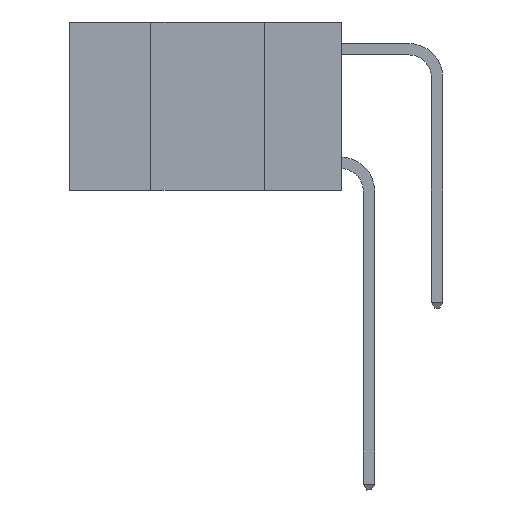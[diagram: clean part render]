
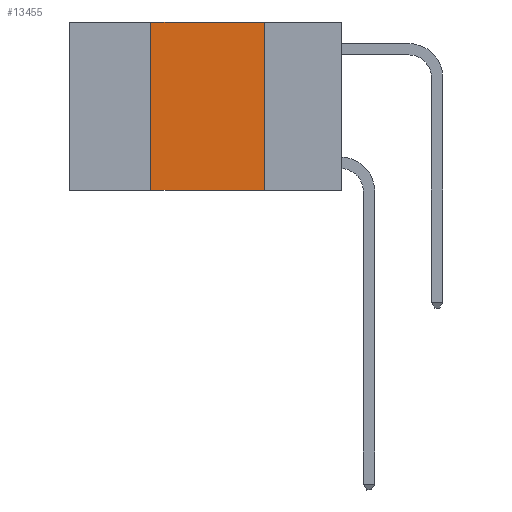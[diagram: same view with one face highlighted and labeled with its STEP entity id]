
A CAD part, left-side view. The second image highlights one B-rep face of the part: STEP entity #13455.
In plain terms, the highlighted planar face has unit normal (-1, 0, 0).
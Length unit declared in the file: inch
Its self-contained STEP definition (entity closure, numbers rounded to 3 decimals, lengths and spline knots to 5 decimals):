
#366 = LINE ( 'NONE', #11684, #16784 ) ;
#1702 = ORIENTED_EDGE ( 'NONE', *, *, #6103, .F. ) ;
#1714 = PLANE ( 'NONE',  #12923 ) ;
#2306 = ORIENTED_EDGE ( 'NONE', *, *, #19817, .F. ) ;
#2364 = CARTESIAN_POINT ( 'NONE',  ( 0., 0.42, -0.37 ) ) ;
#2558 = CARTESIAN_POINT ( 'NONE',  ( 0., 0.6, 0. ) ) ;
#2709 = ORIENTED_EDGE ( 'NONE', *, *, #16716, .F. ) ;
#2812 = VERTEX_POINT ( 'NONE', #15152 ) ;
#2908 = ORIENTED_EDGE ( 'NONE', *, *, #19605, .T. ) ;
#3315 = DIRECTION ( 'NONE',  ( 0., 0., -1. ) ) ;
#3841 = VERTEX_POINT ( 'NONE', #18620 ) ;
#4229 = LINE ( 'NONE', #6850, #16375 ) ;
#4273 = CARTESIAN_POINT ( 'NONE',  ( 0., 0.17, -0.37 ) ) ;
#4730 = FACE_OUTER_BOUND ( 'NONE', #5393, .T. ) ;
#5226 = DIRECTION ( 'NONE',  ( 0., 0., 1. ) ) ;
#5393 = EDGE_LOOP ( 'NONE', ( #1702, #2306, #2709, #2908 ) ) ;
#6103 = EDGE_CURVE ( 'NONE', #3841, #11156, #366, .T. ) ;
#6328 = LINE ( 'NONE', #19474, #17971 ) ;
#6850 = CARTESIAN_POINT ( 'NONE',  ( 0., 0.6, -0.37 ) ) ;
#7567 = VERTEX_POINT ( 'NONE', #2364 ) ;
#11156 = VERTEX_POINT ( 'NONE', #4273 ) ;
#11183 = CARTESIAN_POINT ( 'NONE',  ( 0., 0.6, 0. ) ) ;
#11684 = CARTESIAN_POINT ( 'NONE',  ( 0., 0.17, 0. ) ) ;
#12878 = DIRECTION ( 'NONE',  ( 1., 0., 0. ) ) ;
#12923 = AXIS2_PLACEMENT_3D ( 'NONE', #11183, #12878, #3315 ) ;
#12981 = LINE ( 'NONE', #2558, #13458 ) ;
#13455 = ADVANCED_FACE ( 'NONE', ( #4730 ), #1714, .F. ) ;
#13458 = VECTOR ( 'NONE', #13679, 39.37008 ) ;
#13679 = DIRECTION ( 'NONE',  ( 0., -1., 0. ) ) ;
#14774 = DIRECTION ( 'NONE',  ( 0., -1., 0. ) ) ;
#15152 = CARTESIAN_POINT ( 'NONE',  ( 0., 0.42, 0. ) ) ;
#16375 = VECTOR ( 'NONE', #14774, 39.37008 ) ;
#16716 = EDGE_CURVE ( 'NONE', #7567, #2812, #6328, .T. ) ;
#16784 = VECTOR ( 'NONE', #17916, 39.37008 ) ;
#17916 = DIRECTION ( 'NONE',  ( 0., 0., -1. ) ) ;
#17971 = VECTOR ( 'NONE', #5226, 39.37008 ) ;
#18620 = CARTESIAN_POINT ( 'NONE',  ( 0., 0.17, 0. ) ) ;
#19474 = CARTESIAN_POINT ( 'NONE',  ( 0., 0.42, 0. ) ) ;
#19605 = EDGE_CURVE ( 'NONE', #7567, #11156, #4229, .T. ) ;
#19817 = EDGE_CURVE ( 'NONE', #2812, #3841, #12981, .T. ) ;
